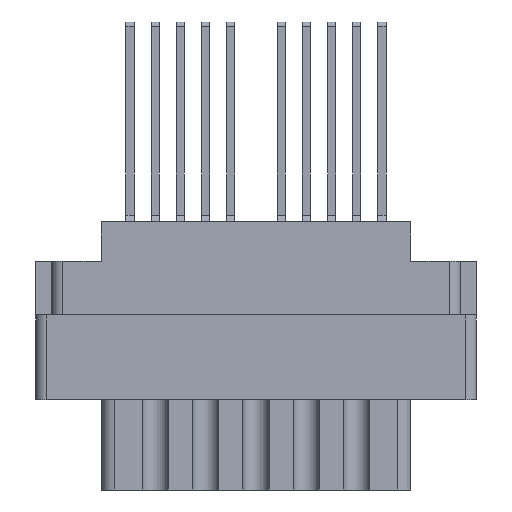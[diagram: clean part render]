
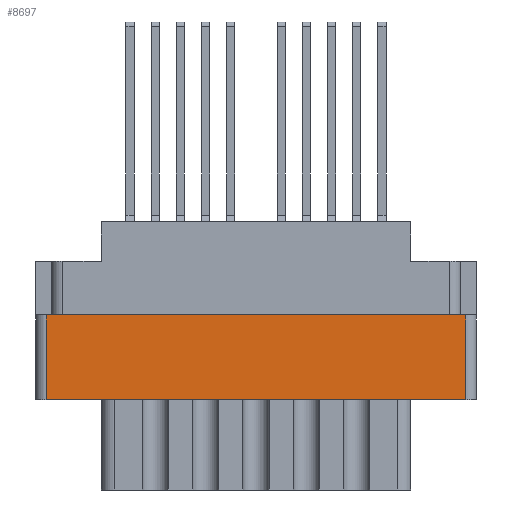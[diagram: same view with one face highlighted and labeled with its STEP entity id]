
A CAD part, front view. The second image highlights one B-rep face of the part: STEP entity #8697.
In plain terms, the highlighted planar face has unit normal (0, -1, 0).
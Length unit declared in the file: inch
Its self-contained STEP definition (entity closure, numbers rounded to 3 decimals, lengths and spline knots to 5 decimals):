
#1248 = VERTEX_POINT ( 'NONE', #21580 ) ;
#2634 = DIRECTION ( 'NONE',  ( 0., 0., 1. ) ) ;
#4086 = EDGE_CURVE ( 'NONE', #1248, #27839, #11417, .T. ) ;
#4751 = CARTESIAN_POINT ( 'NONE',  ( -0.624, -0.343, -0.529 ) ) ;
#5183 = VECTOR ( 'NONE', #8836, 39.37008 ) ;
#6052 = PLANE ( 'NONE',  #8888 ) ;
#7161 = EDGE_CURVE ( 'NONE', #10122, #27839, #9170, .T. ) ;
#7870 = CARTESIAN_POINT ( 'NONE',  ( -0.624, -0.343, -0.798 ) ) ;
#8062 = DIRECTION ( 'NONE',  ( 0., 0., -1. ) ) ;
#8697 = ADVANCED_FACE ( 'NONE', ( #11818 ), #6052, .T. ) ;
#8836 = DIRECTION ( 'NONE',  ( -1., 0., 0. ) ) ;
#8888 = AXIS2_PLACEMENT_3D ( 'NONE', #23207, #27632, #8062 ) ;
#8911 = CARTESIAN_POINT ( 'NONE',  ( 0., -0.343, -0.277 ) ) ;
#9170 = LINE ( 'NONE', #8911, #14304 ) ;
#10122 = VERTEX_POINT ( 'NONE', #19518 ) ;
#10726 = VECTOR ( 'NONE', #2634, 39.37008 ) ;
#11417 = LINE ( 'NONE', #20246, #10726 ) ;
#11818 = FACE_OUTER_BOUND ( 'NONE', #25024, .T. ) ;
#12655 = ORIENTED_EDGE ( 'NONE', *, *, #4086, .T. ) ;
#13397 = LINE ( 'NONE', #7870, #21557 ) ;
#14304 = VECTOR ( 'NONE', #17526, 39.37008 ) ;
#14560 = ORIENTED_EDGE ( 'NONE', *, *, #15763, .T. ) ;
#15525 = EDGE_CURVE ( 'NONE', #1248, #16782, #17512, .T. ) ;
#15763 = EDGE_CURVE ( 'NONE', #10122, #16782, #13397, .T. ) ;
#16782 = VERTEX_POINT ( 'NONE', #4751 ) ;
#17512 = LINE ( 'NONE', #23997, #5183 ) ;
#17526 = DIRECTION ( 'NONE',  ( 1., 0., 0. ) ) ;
#19518 = CARTESIAN_POINT ( 'NONE',  ( -0.624, -0.343, -0.277 ) ) ;
#20246 = CARTESIAN_POINT ( 'NONE',  ( 0.624, -0.343, -0.798 ) ) ;
#21557 = VECTOR ( 'NONE', #27340, 39.37008 ) ;
#21580 = CARTESIAN_POINT ( 'NONE',  ( 0.624, -0.343, -0.529 ) ) ;
#23207 = CARTESIAN_POINT ( 'NONE',  ( -0.656, -0.343, -0.798 ) ) ;
#23997 = CARTESIAN_POINT ( 'NONE',  ( 0., -0.343, -0.529 ) ) ;
#24160 = ORIENTED_EDGE ( 'NONE', *, *, #7161, .F. ) ;
#25024 = EDGE_LOOP ( 'NONE', ( #24160, #14560, #26182, #12655 ) ) ;
#26182 = ORIENTED_EDGE ( 'NONE', *, *, #15525, .F. ) ;
#27340 = DIRECTION ( 'NONE',  ( 0., 0., -1. ) ) ;
#27632 = DIRECTION ( 'NONE',  ( 0., -1., 0. ) ) ;
#27839 = VERTEX_POINT ( 'NONE', #28112 ) ;
#28112 = CARTESIAN_POINT ( 'NONE',  ( 0.624, -0.343, -0.277 ) ) ;
